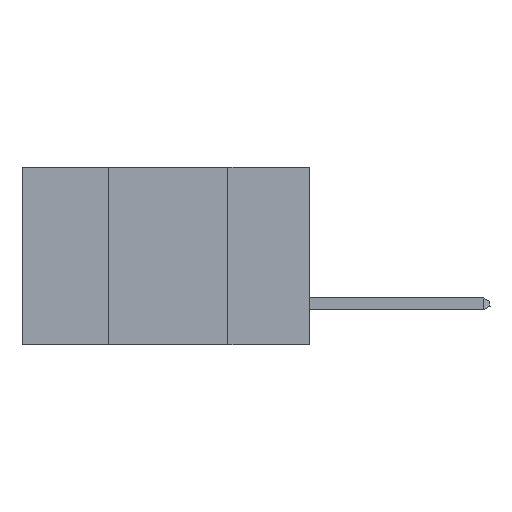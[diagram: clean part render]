
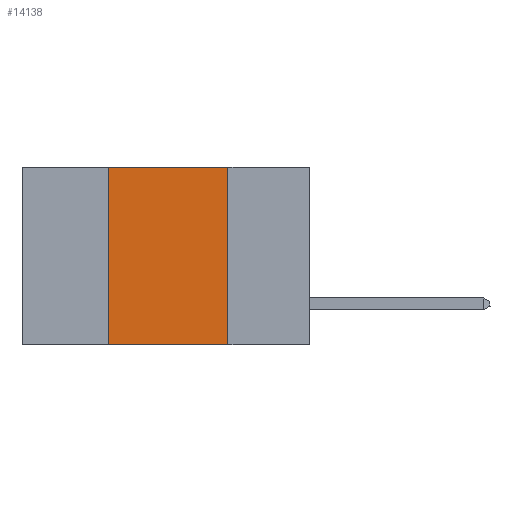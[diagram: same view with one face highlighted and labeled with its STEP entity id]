
A CAD part, left-side view. The second image highlights one B-rep face of the part: STEP entity #14138.
In plain terms, the highlighted planar face has unit normal (-1, 0, 0).
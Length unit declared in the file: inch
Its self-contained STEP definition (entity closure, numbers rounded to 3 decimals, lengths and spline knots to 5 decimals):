
#289 = CARTESIAN_POINT ( 'NONE',  ( 0., 0.6, 0. ) ) ;
#668 = LINE ( 'NONE', #12664, #5671 ) ;
#1092 = VECTOR ( 'NONE', #2287, 39.37008 ) ;
#1243 = CARTESIAN_POINT ( 'NONE',  ( 0., 0.42, 0. ) ) ;
#1388 = DIRECTION ( 'NONE',  ( 1., 0., 0. ) ) ;
#1984 = LINE ( 'NONE', #5902, #1092 ) ;
#2287 = DIRECTION ( 'NONE',  ( 0., 0., 1. ) ) ;
#2333 = CARTESIAN_POINT ( 'NONE',  ( 0., 0.42, -0.37 ) ) ;
#2479 = ORIENTED_EDGE ( 'NONE', *, *, #10292, .F. ) ;
#2569 = PLANE ( 'NONE',  #8605 ) ;
#2794 = DIRECTION ( 'NONE',  ( 0., 0., -1. ) ) ;
#4250 = EDGE_CURVE ( 'NONE', #11049, #4503, #668, .T. ) ;
#4336 = DIRECTION ( 'NONE',  ( 0., 0., -1. ) ) ;
#4503 = VERTEX_POINT ( 'NONE', #6776 ) ;
#5535 = ORIENTED_EDGE ( 'NONE', *, *, #15456, .F. ) ;
#5671 = VECTOR ( 'NONE', #9382, 39.37008 ) ;
#5902 = CARTESIAN_POINT ( 'NONE',  ( 0., 0.42, 0. ) ) ;
#6711 = CARTESIAN_POINT ( 'NONE',  ( 0., 0.17, 0. ) ) ;
#6776 = CARTESIAN_POINT ( 'NONE',  ( 0., 0.17, 0. ) ) ;
#6843 = LINE ( 'NONE', #15353, #8662 ) ;
#7738 = EDGE_LOOP ( 'NONE', ( #2479, #8792, #5535, #9364 ) ) ;
#7781 = EDGE_CURVE ( 'NONE', #12756, #12502, #6843, .T. ) ;
#7898 = VECTOR ( 'NONE', #4336, 39.37008 ) ;
#8605 = AXIS2_PLACEMENT_3D ( 'NONE', #289, #1388, #2794 ) ;
#8662 = VECTOR ( 'NONE', #11597, 39.37008 ) ;
#8792 = ORIENTED_EDGE ( 'NONE', *, *, #4250, .F. ) ;
#9364 = ORIENTED_EDGE ( 'NONE', *, *, #7781, .T. ) ;
#9382 = DIRECTION ( 'NONE',  ( 0., -1., 0. ) ) ;
#10292 = EDGE_CURVE ( 'NONE', #4503, #12502, #12728, .T. ) ;
#11049 = VERTEX_POINT ( 'NONE', #1243 ) ;
#11597 = DIRECTION ( 'NONE',  ( 0., -1., 0. ) ) ;
#12146 = CARTESIAN_POINT ( 'NONE',  ( 0., 0.17, -0.37 ) ) ;
#12502 = VERTEX_POINT ( 'NONE', #12146 ) ;
#12664 = CARTESIAN_POINT ( 'NONE',  ( 0., 0.6, 0. ) ) ;
#12728 = LINE ( 'NONE', #6711, #7898 ) ;
#12756 = VERTEX_POINT ( 'NONE', #2333 ) ;
#14138 = ADVANCED_FACE ( 'NONE', ( #14558 ), #2569, .F. ) ;
#14558 = FACE_OUTER_BOUND ( 'NONE', #7738, .T. ) ;
#15353 = CARTESIAN_POINT ( 'NONE',  ( 0., 0.6, -0.37 ) ) ;
#15456 = EDGE_CURVE ( 'NONE', #12756, #11049, #1984, .T. ) ;
